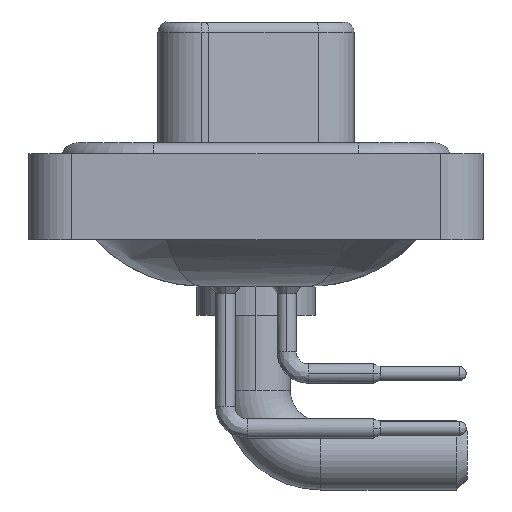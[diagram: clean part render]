
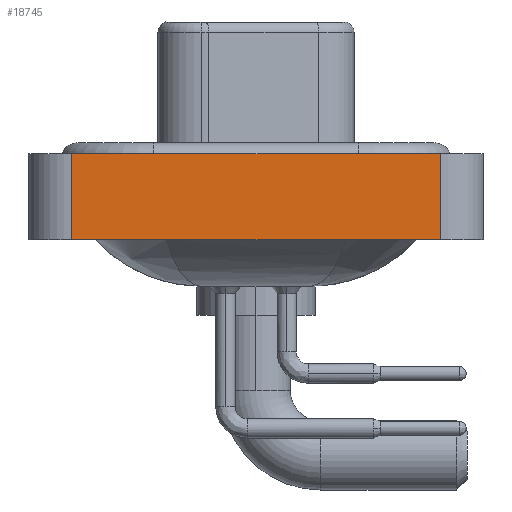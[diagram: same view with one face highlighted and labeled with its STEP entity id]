
A CAD part, left-side view. The second image highlights one B-rep face of the part: STEP entity #18745.
In plain terms, the highlighted planar face has unit normal (-1, 0, 0).
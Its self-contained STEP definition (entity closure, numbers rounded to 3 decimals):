
#1361 = CARTESIAN_POINT ( 'NONE',  ( -7.3, -8.55, -3.6 ) ) ;
#4535 = VECTOR ( 'NONE', #6531, 1000. ) ;
#5306 = DIRECTION ( 'NONE',  ( 0., 0., 1. ) ) ;
#5333 = EDGE_LOOP ( 'NONE', ( #14977, #16864, #21297, #14424 ) ) ;
#5923 = LINE ( 'NONE', #9874, #6177 ) ;
#6177 = VECTOR ( 'NONE', #22091, 1000. ) ;
#6531 = DIRECTION ( 'NONE',  ( 0., -1., 0. ) ) ;
#7279 = FACE_OUTER_BOUND ( 'NONE', #5333, .T. ) ;
#8613 = CARTESIAN_POINT ( 'NONE',  ( -7.3, 8.55, 0.4 ) ) ;
#9874 = CARTESIAN_POINT ( 'NONE',  ( -7.3, -8.55, -3.6 ) ) ;
#10597 = CARTESIAN_POINT ( 'NONE',  ( -7.3, 8.55, -3.6 ) ) ;
#10632 = AXIS2_PLACEMENT_3D ( 'NONE', #1361, #23315, #5306 ) ;
#11620 = DIRECTION ( 'NONE',  ( 0., -1., 0. ) ) ;
#12741 = CARTESIAN_POINT ( 'NONE',  ( -7.3, -8.55, -3.6 ) ) ;
#13696 = LINE ( 'NONE', #21436, #20954 ) ;
#14424 = ORIENTED_EDGE ( 'NONE', *, *, #22003, .T. ) ;
#14434 = LINE ( 'NONE', #12741, #4535 ) ;
#14977 = ORIENTED_EDGE ( 'NONE', *, *, #24461, .T. ) ;
#15260 = CARTESIAN_POINT ( 'NONE',  ( -7.3, -8.55, -3.6 ) ) ;
#15287 = LINE ( 'NONE', #17383, #19754 ) ;
#15303 = PLANE ( 'NONE',  #10632 ) ;
#15782 = EDGE_CURVE ( 'NONE', #16986, #18780, #15287, .T. ) ;
#16830 = VERTEX_POINT ( 'NONE', #10597 ) ;
#16864 = ORIENTED_EDGE ( 'NONE', *, *, #15782, .F. ) ;
#16986 = VERTEX_POINT ( 'NONE', #8613 ) ;
#17383 = CARTESIAN_POINT ( 'NONE',  ( -7.3, -8.55, 0.4 ) ) ;
#18745 = ADVANCED_FACE ( 'NONE', ( #7279 ), #15303, .T. ) ;
#18780 = VERTEX_POINT ( 'NONE', #25702 ) ;
#19754 = VECTOR ( 'NONE', #11620, 1000. ) ;
#20954 = VECTOR ( 'NONE', #21694, 1000. ) ;
#21167 = VERTEX_POINT ( 'NONE', #15260 ) ;
#21297 = ORIENTED_EDGE ( 'NONE', *, *, #23596, .F. ) ;
#21436 = CARTESIAN_POINT ( 'NONE',  ( -7.3, 8.55, -3.6 ) ) ;
#21694 = DIRECTION ( 'NONE',  ( 0., 0., 1. ) ) ;
#22003 = EDGE_CURVE ( 'NONE', #16830, #21167, #14434, .T. ) ;
#22091 = DIRECTION ( 'NONE',  ( 0., 0., 1. ) ) ;
#23315 = DIRECTION ( 'NONE',  ( -1., 0., 0. ) ) ;
#23596 = EDGE_CURVE ( 'NONE', #16830, #16986, #13696, .T. ) ;
#24461 = EDGE_CURVE ( 'NONE', #21167, #18780, #5923, .T. ) ;
#25702 = CARTESIAN_POINT ( 'NONE',  ( -7.3, -8.55, 0.4 ) ) ;
